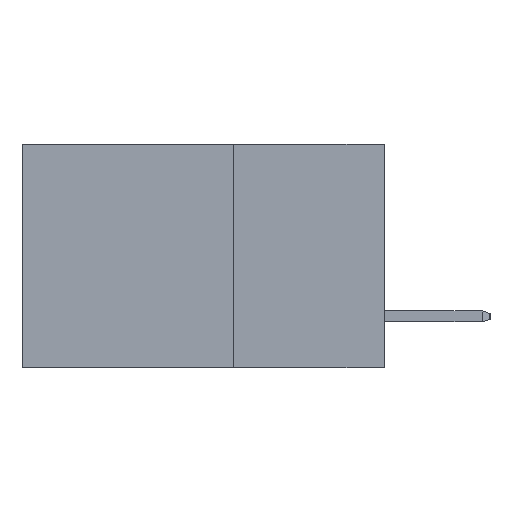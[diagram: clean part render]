
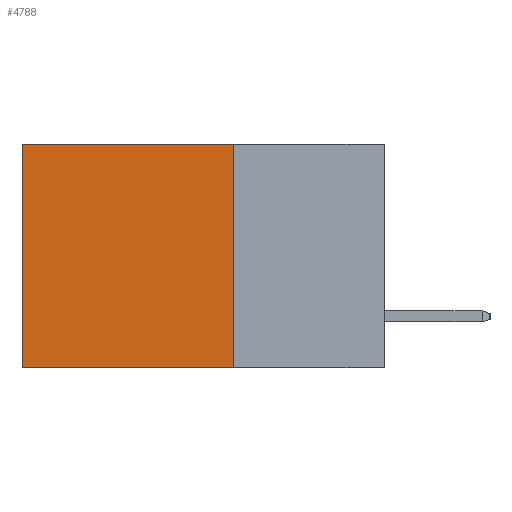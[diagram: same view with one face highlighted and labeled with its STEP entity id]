
A CAD part, left-side view. The second image highlights one B-rep face of the part: STEP entity #4788.
In plain terms, the highlighted planar face has unit normal (-1, 0, 0).
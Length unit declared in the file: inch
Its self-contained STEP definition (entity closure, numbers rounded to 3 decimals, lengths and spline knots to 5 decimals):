
#190 = EDGE_LOOP ( 'NONE', ( #13467, #14035, #12121, #15913 ) ) ;
#194 = DIRECTION ( 'NONE',  ( 0., 1., 0. ) ) ;
#866 = EDGE_CURVE ( 'NONE', #7673, #8639, #5950, .T. ) ;
#1543 = VECTOR ( 'NONE', #12152, 39.37008 ) ;
#1753 = EDGE_CURVE ( 'NONE', #3971, #8639, #8602, .T. ) ;
#2178 = CARTESIAN_POINT ( 'NONE',  ( 0.298, 0.6, 0. ) ) ;
#3925 = CARTESIAN_POINT ( 'NONE',  ( 0.298, 0.25, 0. ) ) ;
#3971 = VERTEX_POINT ( 'NONE', #12674 ) ;
#3981 = PLANE ( 'NONE',  #5045 ) ;
#4532 = DIRECTION ( 'NONE',  ( 0., 1., 0. ) ) ;
#4788 = ADVANCED_FACE ( 'NONE', ( #19851 ), #3981, .F. ) ;
#4988 = EDGE_CURVE ( 'NONE', #14597, #7673, #16786, .T. ) ;
#5045 = AXIS2_PLACEMENT_3D ( 'NONE', #3925, #9417, #9413 ) ;
#5577 = VECTOR ( 'NONE', #11971, 39.37008 ) ;
#5950 = LINE ( 'NONE', #15075, #1543 ) ;
#7673 = VERTEX_POINT ( 'NONE', #2178 ) ;
#8095 = CARTESIAN_POINT ( 'NONE',  ( 0.298, 0.25, 0. ) ) ;
#8571 = CARTESIAN_POINT ( 'NONE',  ( 0.298, 0.6, -0.37 ) ) ;
#8602 = LINE ( 'NONE', #12568, #16981 ) ;
#8639 = VERTEX_POINT ( 'NONE', #8571 ) ;
#9413 = DIRECTION ( 'NONE',  ( 0., 0., -1. ) ) ;
#9417 = DIRECTION ( 'NONE',  ( 1., 0., 0. ) ) ;
#10093 = LINE ( 'NONE', #10290, #5577 ) ;
#10290 = CARTESIAN_POINT ( 'NONE',  ( 0.298, 0.25, 0. ) ) ;
#11266 = EDGE_CURVE ( 'NONE', #14597, #3971, #10093, .T. ) ;
#11971 = DIRECTION ( 'NONE',  ( 0., 0., -1. ) ) ;
#12121 = ORIENTED_EDGE ( 'NONE', *, *, #11266, .F. ) ;
#12152 = DIRECTION ( 'NONE',  ( 0., 0., -1. ) ) ;
#12568 = CARTESIAN_POINT ( 'NONE',  ( 0.298, 0.25, -0.37 ) ) ;
#12674 = CARTESIAN_POINT ( 'NONE',  ( 0.298, 0.25, -0.37 ) ) ;
#13467 = ORIENTED_EDGE ( 'NONE', *, *, #866, .T. ) ;
#14035 = ORIENTED_EDGE ( 'NONE', *, *, #1753, .F. ) ;
#14597 = VERTEX_POINT ( 'NONE', #8095 ) ;
#15075 = CARTESIAN_POINT ( 'NONE',  ( 0.298, 0.6, 0. ) ) ;
#15913 = ORIENTED_EDGE ( 'NONE', *, *, #4988, .T. ) ;
#16786 = LINE ( 'NONE', #17171, #19280 ) ;
#16981 = VECTOR ( 'NONE', #194, 39.37008 ) ;
#17171 = CARTESIAN_POINT ( 'NONE',  ( 0.298, 0.25, 0. ) ) ;
#19280 = VECTOR ( 'NONE', #4532, 39.37008 ) ;
#19851 = FACE_OUTER_BOUND ( 'NONE', #190, .T. ) ;
